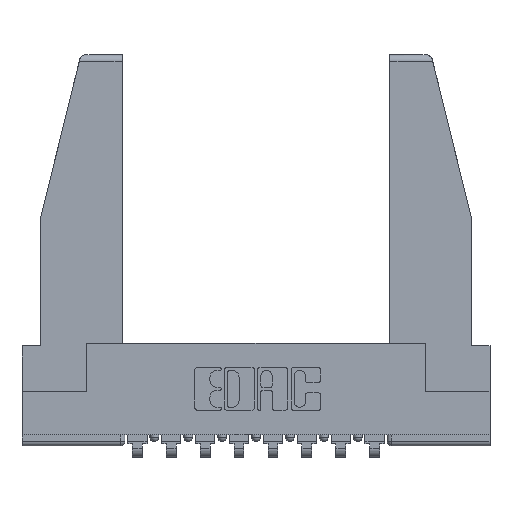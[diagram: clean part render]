
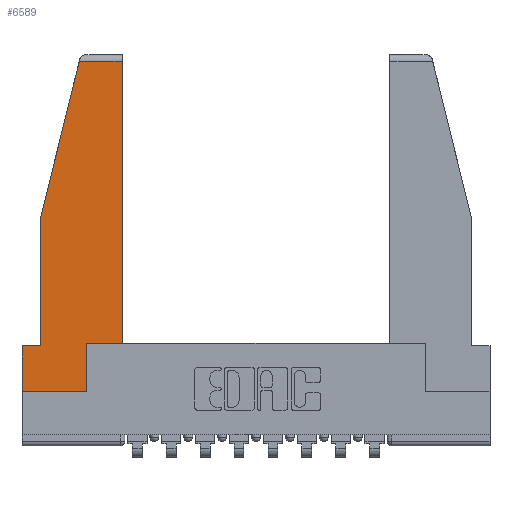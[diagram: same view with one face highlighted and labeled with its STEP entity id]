
A CAD part, top view. The second image highlights one B-rep face of the part: STEP entity #6589.
In plain terms, the highlighted planar face has unit normal (0, 0, 1).
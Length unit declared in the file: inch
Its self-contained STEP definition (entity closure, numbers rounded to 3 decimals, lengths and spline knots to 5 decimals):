
#53 = ORIENTED_EDGE ( 'NONE', *, *, #5173, .T. ) ;
#77 = ORIENTED_EDGE ( 'NONE', *, *, #10450, .T. ) ;
#136 = VECTOR ( 'NONE', #11021, 39.37008 ) ;
#173 = ORIENTED_EDGE ( 'NONE', *, *, #10740, .T. ) ;
#355 = CARTESIAN_POINT ( 'NONE',  ( 0., 0., 0. ) ) ;
#361 = DIRECTION ( 'NONE',  ( 0., 1., 0. ) ) ;
#505 = CARTESIAN_POINT ( 'NONE',  ( 0.297, 0., 0. ) ) ;
#1121 = DIRECTION ( 'NONE',  ( 0., -1., 0. ) ) ;
#1151 = EDGE_CURVE ( 'NONE', #9808, #12922, #13687, .T. ) ;
#1191 = VECTOR ( 'NONE', #13539, 39.37008 ) ;
#1248 = LINE ( 'NONE', #2115, #6960 ) ;
#1577 = DIRECTION ( 'NONE',  ( 1., 0., 0. ) ) ;
#1617 = PLANE ( 'NONE',  #14144 ) ;
#2043 = DIRECTION ( 'NONE',  ( -1., 0., 0. ) ) ;
#2115 = CARTESIAN_POINT ( 'NONE',  ( 0., 0., 0. ) ) ;
#2208 = DIRECTION ( 'NONE',  ( 1., 0., 0. ) ) ;
#2403 = LINE ( 'NONE', #9232, #5859 ) ;
#2565 = CARTESIAN_POINT ( 'NONE',  ( 0.461, 0.223, 0. ) ) ;
#3103 = VECTOR ( 'NONE', #9285, 39.37008 ) ;
#3174 = ORIENTED_EDGE ( 'NONE', *, *, #1151, .T. ) ;
#3345 = LINE ( 'NONE', #505, #13386 ) ;
#3700 = CARTESIAN_POINT ( 'NONE',  ( 0.086, 0.21, 0. ) ) ;
#4348 = CARTESIAN_POINT ( 'NONE',  ( 0., 0.21, 0. ) ) ;
#4363 = CARTESIAN_POINT ( 'NONE',  ( 0.2636, 1.52, 0. ) ) ;
#4836 = VECTOR ( 'NONE', #7219, 39.37008 ) ;
#4911 = CARTESIAN_POINT ( 'NONE',  ( 0., 1.52, 0. ) ) ;
#5071 = CARTESIAN_POINT ( 'NONE',  ( 0.297, 0.223, 0. ) ) ;
#5085 = ORIENTED_EDGE ( 'NONE', *, *, #9622, .T. ) ;
#5173 = EDGE_CURVE ( 'NONE', #6016, #9808, #6036, .T. ) ;
#5859 = VECTOR ( 'NONE', #10849, 39.37008 ) ;
#6016 = VERTEX_POINT ( 'NONE', #6473 ) ;
#6036 = LINE ( 'NONE', #2565, #3103 ) ;
#6076 = EDGE_CURVE ( 'NONE', #13453, #6016, #2403, .T. ) ;
#6473 = CARTESIAN_POINT ( 'NONE',  ( 0.461, 0.223, 0. ) ) ;
#6494 = CARTESIAN_POINT ( 'NONE',  ( 0., 0.21, 0. ) ) ;
#6589 = ADVANCED_FACE ( 'NONE', ( #9991 ), #1617, .T. ) ;
#6960 = VECTOR ( 'NONE', #2208, 39.37008 ) ;
#7038 = VERTEX_POINT ( 'NONE', #3700 ) ;
#7219 = DIRECTION ( 'NONE',  ( -1., 0., 0. ) ) ;
#7640 = CARTESIAN_POINT ( 'NONE',  ( 0.086, 0.8, 0. ) ) ;
#8000 = CARTESIAN_POINT ( 'NONE',  ( 0.461, 1.52, 0. ) ) ;
#8201 = CARTESIAN_POINT ( 'NONE',  ( 0., 0., 0. ) ) ;
#8296 = DIRECTION ( 'NONE',  ( 0., 0., 1. ) ) ;
#8348 = ORIENTED_EDGE ( 'NONE', *, *, #11730, .T. ) ;
#8493 = EDGE_LOOP ( 'NONE', ( #53, #3174, #173, #14140, #5085, #77, #8348, #11467, #10830 ) ) ;
#8842 = LINE ( 'NONE', #11508, #1191 ) ;
#9036 = CARTESIAN_POINT ( 'NONE',  ( 0., 0.21, 0. ) ) ;
#9232 = CARTESIAN_POINT ( 'NONE',  ( 0.297, 0.223, 0. ) ) ;
#9285 = DIRECTION ( 'NONE',  ( 0., 1., 0. ) ) ;
#9622 = EDGE_CURVE ( 'NONE', #7038, #13663, #13641, .T. ) ;
#9808 = VERTEX_POINT ( 'NONE', #8000 ) ;
#9991 = FACE_OUTER_BOUND ( 'NONE', #8493, .T. ) ;
#10450 = EDGE_CURVE ( 'NONE', #13663, #11863, #14349, .T. ) ;
#10740 = EDGE_CURVE ( 'NONE', #12922, #12959, #8842, .T. ) ;
#10830 = ORIENTED_EDGE ( 'NONE', *, *, #6076, .T. ) ;
#10849 = DIRECTION ( 'NONE',  ( 1., 0., 0. ) ) ;
#10922 = LINE ( 'NONE', #7640, #11971 ) ;
#10967 = CARTESIAN_POINT ( 'NONE',  ( 0.297, 0., 0. ) ) ;
#11021 = DIRECTION ( 'NONE',  ( 0., -1., 0. ) ) ;
#11467 = ORIENTED_EDGE ( 'NONE', *, *, #11485, .T. ) ;
#11485 = EDGE_CURVE ( 'NONE', #11963, #13453, #3345, .T. ) ;
#11508 = CARTESIAN_POINT ( 'NONE',  ( 0.271, 1.55, 0. ) ) ;
#11730 = EDGE_CURVE ( 'NONE', #11863, #11963, #1248, .T. ) ;
#11863 = VERTEX_POINT ( 'NONE', #355 ) ;
#11963 = VERTEX_POINT ( 'NONE', #10967 ) ;
#11971 = VECTOR ( 'NONE', #1121, 39.37008 ) ;
#12922 = VERTEX_POINT ( 'NONE', #4363 ) ;
#12959 = VERTEX_POINT ( 'NONE', #13236 ) ;
#13005 = EDGE_CURVE ( 'NONE', #12959, #7038, #10922, .T. ) ;
#13104 = VECTOR ( 'NONE', #2043, 39.37008 ) ;
#13236 = CARTESIAN_POINT ( 'NONE',  ( 0.086, 0.8, 0. ) ) ;
#13386 = VECTOR ( 'NONE', #361, 39.37008 ) ;
#13453 = VERTEX_POINT ( 'NONE', #5071 ) ;
#13539 = DIRECTION ( 'NONE',  ( -0.239, -0.971, 0. ) ) ;
#13641 = LINE ( 'NONE', #6494, #13104 ) ;
#13663 = VERTEX_POINT ( 'NONE', #4348 ) ;
#13687 = LINE ( 'NONE', #4911, #4836 ) ;
#14140 = ORIENTED_EDGE ( 'NONE', *, *, #13005, .T. ) ;
#14144 = AXIS2_PLACEMENT_3D ( 'NONE', #8201, #8296, #1577 ) ;
#14349 = LINE ( 'NONE', #9036, #136 ) ;
